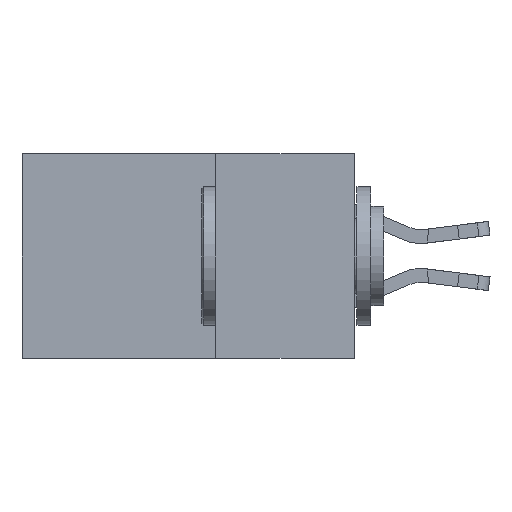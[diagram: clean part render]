
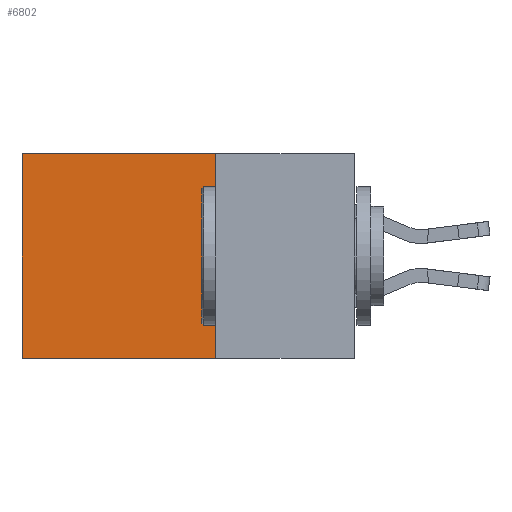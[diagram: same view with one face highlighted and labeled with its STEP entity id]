
A CAD part, left-side view. The second image highlights one B-rep face of the part: STEP entity #6802.
In plain terms, the highlighted planar face has unit normal (-1, 0, 0).
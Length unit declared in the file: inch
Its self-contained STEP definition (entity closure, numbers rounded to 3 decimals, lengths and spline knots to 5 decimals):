
#963 = ORIENTED_EDGE ( 'NONE', *, *, #16536, .F. ) ;
#2099 = FACE_OUTER_BOUND ( 'NONE', #3386, .T. ) ;
#2788 = LINE ( 'NONE', #10420, #18974 ) ;
#2880 = CARTESIAN_POINT ( 'NONE',  ( 0.2615, 0.6, 0. ) ) ;
#3386 = EDGE_LOOP ( 'NONE', ( #15329, #7196, #963, #7140 ) ) ;
#3422 = DIRECTION ( 'NONE',  ( 1., 0., 0. ) ) ;
#4090 = CARTESIAN_POINT ( 'NONE',  ( 0.2615, 0.25, -0.37 ) ) ;
#4164 = DIRECTION ( 'NONE',  ( 0., 0., -1. ) ) ;
#4637 = EDGE_CURVE ( 'NONE', #16666, #15840, #16976, .T. ) ;
#5618 = VERTEX_POINT ( 'NONE', #6949 ) ;
#6388 = CARTESIAN_POINT ( 'NONE',  ( 0.2615, 0.25, 0. ) ) ;
#6753 = LINE ( 'NONE', #13889, #14144 ) ;
#6802 = ADVANCED_FACE ( 'NONE', ( #2099 ), #12810, .F. ) ;
#6949 = CARTESIAN_POINT ( 'NONE',  ( 0.2615, 0.25, -0.37 ) ) ;
#7140 = ORIENTED_EDGE ( 'NONE', *, *, #4637, .T. ) ;
#7196 = ORIENTED_EDGE ( 'NONE', *, *, #11578, .F. ) ;
#10420 = CARTESIAN_POINT ( 'NONE',  ( 0.2615, 0.6, -0.37 ) ) ;
#10754 = DIRECTION ( 'NONE',  ( 0., 1., 0. ) ) ;
#10853 = CARTESIAN_POINT ( 'NONE',  ( 0.2615, 0.25, 0. ) ) ;
#11488 = VECTOR ( 'NONE', #15146, 39.37008 ) ;
#11578 = EDGE_CURVE ( 'NONE', #5618, #13886, #11990, .T. ) ;
#11990 = LINE ( 'NONE', #4090, #11488 ) ;
#12810 = PLANE ( 'NONE',  #15784 ) ;
#13886 = VERTEX_POINT ( 'NONE', #13953 ) ;
#13889 = CARTESIAN_POINT ( 'NONE',  ( 0.2615, 0.25, -0.37 ) ) ;
#13953 = CARTESIAN_POINT ( 'NONE',  ( 0.2615, 0.6, -0.37 ) ) ;
#14144 = VECTOR ( 'NONE', #18608, 39.37008 ) ;
#14394 = DIRECTION ( 'NONE',  ( 0., 0., -1. ) ) ;
#15146 = DIRECTION ( 'NONE',  ( 0., 1., 0. ) ) ;
#15329 = ORIENTED_EDGE ( 'NONE', *, *, #18035, .T. ) ;
#15784 = AXIS2_PLACEMENT_3D ( 'NONE', #19050, #3422, #14394 ) ;
#15840 = VERTEX_POINT ( 'NONE', #2880 ) ;
#16536 = EDGE_CURVE ( 'NONE', #16666, #5618, #6753, .T. ) ;
#16666 = VERTEX_POINT ( 'NONE', #6388 ) ;
#16976 = LINE ( 'NONE', #10853, #20151 ) ;
#18035 = EDGE_CURVE ( 'NONE', #15840, #13886, #2788, .T. ) ;
#18608 = DIRECTION ( 'NONE',  ( 0., 0., -1. ) ) ;
#18974 = VECTOR ( 'NONE', #4164, 39.37008 ) ;
#19050 = CARTESIAN_POINT ( 'NONE',  ( 0.2615, 0.25, -0.37 ) ) ;
#20151 = VECTOR ( 'NONE', #10754, 39.37008 ) ;
